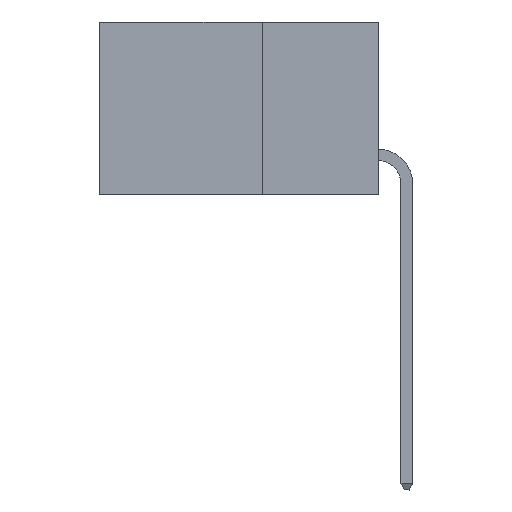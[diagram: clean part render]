
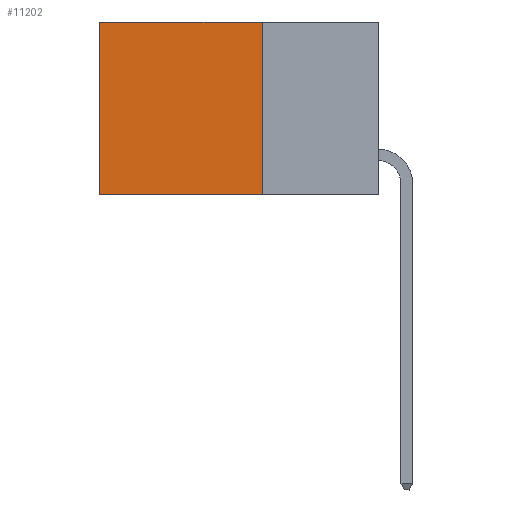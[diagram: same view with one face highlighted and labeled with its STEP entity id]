
A CAD part, left-side view. The second image highlights one B-rep face of the part: STEP entity #11202.
In plain terms, the highlighted planar face has unit normal (-1, 0, 0).
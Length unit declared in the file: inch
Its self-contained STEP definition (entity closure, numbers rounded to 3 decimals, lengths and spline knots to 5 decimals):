
#569 = LINE ( 'NONE', #1914, #4819 ) ;
#959 = VERTEX_POINT ( 'NONE', #14967 ) ;
#1671 = VERTEX_POINT ( 'NONE', #9877 ) ;
#1789 = DIRECTION ( 'NONE',  ( 0., 1., 0. ) ) ;
#1914 = CARTESIAN_POINT ( 'NONE',  ( 0.298, 0.6, 0. ) ) ;
#2349 = EDGE_CURVE ( 'NONE', #12941, #1671, #569, .T. ) ;
#2549 = DIRECTION ( 'NONE',  ( 0., 1., 0. ) ) ;
#2806 = AXIS2_PLACEMENT_3D ( 'NONE', #12750, #16800, #14311 ) ;
#3336 = EDGE_CURVE ( 'NONE', #13241, #959, #3876, .T. ) ;
#3876 = LINE ( 'NONE', #9773, #17396 ) ;
#4819 = VECTOR ( 'NONE', #13313, 39.37008 ) ;
#5222 = FACE_OUTER_BOUND ( 'NONE', #10668, .T. ) ;
#5674 = PLANE ( 'NONE',  #2806 ) ;
#6898 = ORIENTED_EDGE ( 'NONE', *, *, #17549, .T. ) ;
#6913 = ORIENTED_EDGE ( 'NONE', *, *, #3336, .F. ) ;
#7020 = DIRECTION ( 'NONE',  ( 0., 0., -1. ) ) ;
#7680 = VECTOR ( 'NONE', #1789, 39.37008 ) ;
#7706 = CARTESIAN_POINT ( 'NONE',  ( 0.298, 0.6, 0. ) ) ;
#8162 = EDGE_CURVE ( 'NONE', #959, #1671, #17729, .T. ) ;
#9749 = VECTOR ( 'NONE', #2549, 39.37008 ) ;
#9773 = CARTESIAN_POINT ( 'NONE',  ( 0.298, 0.25, 0. ) ) ;
#9877 = CARTESIAN_POINT ( 'NONE',  ( 0.298, 0.6, -0.37 ) ) ;
#10457 = CARTESIAN_POINT ( 'NONE',  ( 0.298, 0.25, 0. ) ) ;
#10668 = EDGE_LOOP ( 'NONE', ( #12214, #13633, #6913, #6898 ) ) ;
#11202 = ADVANCED_FACE ( 'NONE', ( #5222 ), #5674, .F. ) ;
#11440 = LINE ( 'NONE', #10457, #7680 ) ;
#12214 = ORIENTED_EDGE ( 'NONE', *, *, #2349, .T. ) ;
#12750 = CARTESIAN_POINT ( 'NONE',  ( 0.298, 0.25, 0. ) ) ;
#12941 = VERTEX_POINT ( 'NONE', #7706 ) ;
#13005 = CARTESIAN_POINT ( 'NONE',  ( 0.298, 0.25, 0. ) ) ;
#13241 = VERTEX_POINT ( 'NONE', #13005 ) ;
#13313 = DIRECTION ( 'NONE',  ( 0., 0., -1. ) ) ;
#13633 = ORIENTED_EDGE ( 'NONE', *, *, #8162, .F. ) ;
#13892 = CARTESIAN_POINT ( 'NONE',  ( 0.298, 0.25, -0.37 ) ) ;
#14311 = DIRECTION ( 'NONE',  ( 0., 0., -1. ) ) ;
#14967 = CARTESIAN_POINT ( 'NONE',  ( 0.298, 0.25, -0.37 ) ) ;
#16800 = DIRECTION ( 'NONE',  ( 1., 0., 0. ) ) ;
#17396 = VECTOR ( 'NONE', #7020, 39.37008 ) ;
#17549 = EDGE_CURVE ( 'NONE', #13241, #12941, #11440, .T. ) ;
#17729 = LINE ( 'NONE', #13892, #9749 ) ;
